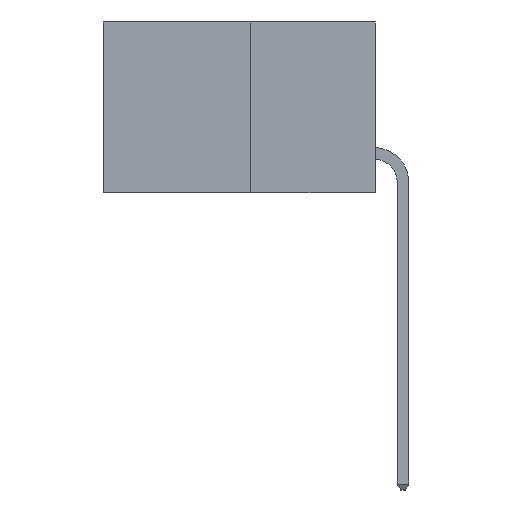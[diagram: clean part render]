
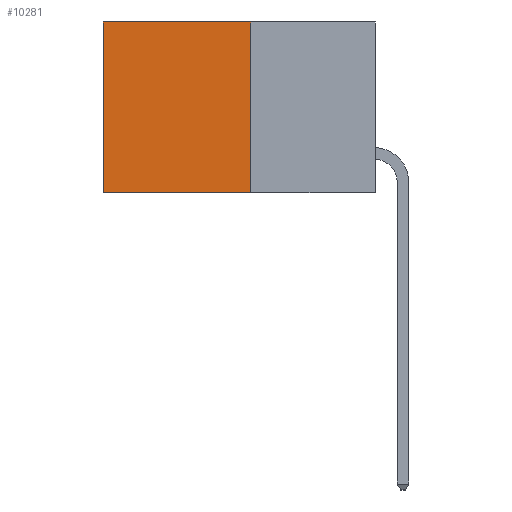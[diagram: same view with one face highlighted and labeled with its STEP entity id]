
A CAD part, left-side view. The second image highlights one B-rep face of the part: STEP entity #10281.
In plain terms, the highlighted planar face has unit normal (-1, 0, 0).
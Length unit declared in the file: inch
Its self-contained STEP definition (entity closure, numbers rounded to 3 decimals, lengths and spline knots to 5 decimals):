
#390 = VECTOR ( 'NONE', #3709, 39.37008 ) ;
#1493 = DIRECTION ( 'NONE',  ( 0., 0., -1. ) ) ;
#2143 = LINE ( 'NONE', #10936, #10471 ) ;
#2756 = ORIENTED_EDGE ( 'NONE', *, *, #12420, .T. ) ;
#2822 = ORIENTED_EDGE ( 'NONE', *, *, #12268, .F. ) ;
#2849 = VERTEX_POINT ( 'NONE', #3925 ) ;
#3188 = ORIENTED_EDGE ( 'NONE', *, *, #12290, .F. ) ;
#3709 = DIRECTION ( 'NONE',  ( 0., 1., 0. ) ) ;
#3925 = CARTESIAN_POINT ( 'NONE',  ( 0.277, 0.27, 0. ) ) ;
#4237 = ORIENTED_EDGE ( 'NONE', *, *, #12315, .T. ) ;
#5152 = PLANE ( 'NONE',  #10044 ) ;
#5187 = DIRECTION ( 'NONE',  ( 0., 0., -1. ) ) ;
#5719 = VERTEX_POINT ( 'NONE', #10018 ) ;
#5939 = VERTEX_POINT ( 'NONE', #15003 ) ;
#6303 = CARTESIAN_POINT ( 'NONE',  ( 0.277, 0.27, -0.37 ) ) ;
#6981 = LINE ( 'NONE', #10806, #11891 ) ;
#8000 = VERTEX_POINT ( 'NONE', #8934 ) ;
#8774 = DIRECTION ( 'NONE',  ( 1., 0., 0. ) ) ;
#8934 = CARTESIAN_POINT ( 'NONE',  ( 0.277, 0.59, 0. ) ) ;
#9297 = VECTOR ( 'NONE', #12994, 39.37008 ) ;
#9618 = CARTESIAN_POINT ( 'NONE',  ( 0.277, 0.27, -0.37 ) ) ;
#9666 = CARTESIAN_POINT ( 'NONE',  ( 0.277, 0.27, -0.37 ) ) ;
#9693 = EDGE_LOOP ( 'NONE', ( #2756, #2822, #3188, #4237 ) ) ;
#10018 = CARTESIAN_POINT ( 'NONE',  ( 0.277, 0.27, -0.37 ) ) ;
#10044 = AXIS2_PLACEMENT_3D ( 'NONE', #6303, #8774, #1493 ) ;
#10281 = ADVANCED_FACE ( 'NONE', ( #11749 ), #5152, .F. ) ;
#10471 = VECTOR ( 'NONE', #5187, 39.37008 ) ;
#10806 = CARTESIAN_POINT ( 'NONE',  ( 0.277, 0.27, 0. ) ) ;
#10936 = CARTESIAN_POINT ( 'NONE',  ( 0.277, 0.59, -0.37 ) ) ;
#11749 = FACE_OUTER_BOUND ( 'NONE', #9693, .T. ) ;
#11891 = VECTOR ( 'NONE', #11945, 39.37008 ) ;
#11945 = DIRECTION ( 'NONE',  ( 0., 1., 0. ) ) ;
#12238 = LINE ( 'NONE', #9666, #9297 ) ;
#12268 = EDGE_CURVE ( 'NONE', #5719, #5939, #13251, .T. ) ;
#12290 = EDGE_CURVE ( 'NONE', #2849, #5719, #12238, .T. ) ;
#12315 = EDGE_CURVE ( 'NONE', #2849, #8000, #6981, .T. ) ;
#12420 = EDGE_CURVE ( 'NONE', #8000, #5939, #2143, .T. ) ;
#12994 = DIRECTION ( 'NONE',  ( 0., 0., -1. ) ) ;
#13251 = LINE ( 'NONE', #9618, #390 ) ;
#15003 = CARTESIAN_POINT ( 'NONE',  ( 0.277, 0.59, -0.37 ) ) ;
